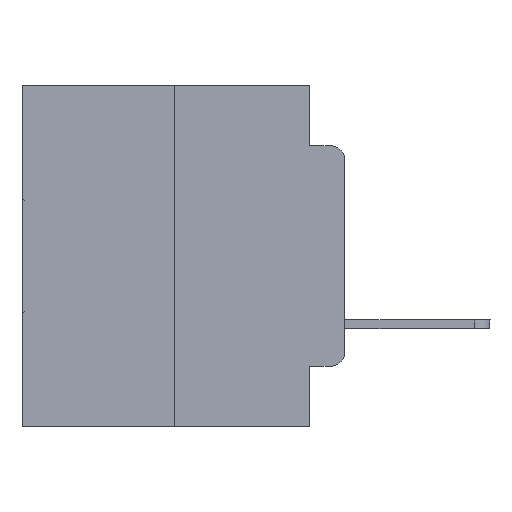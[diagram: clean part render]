
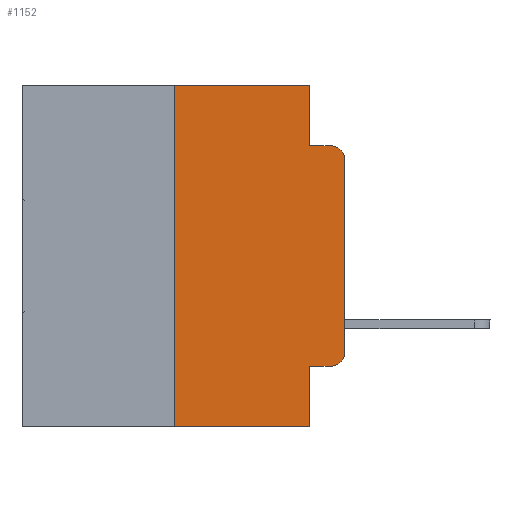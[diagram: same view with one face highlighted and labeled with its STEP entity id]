
A CAD part, left-side view. The second image highlights one B-rep face of the part: STEP entity #1152.
In plain terms, the highlighted planar face has unit normal (-1, 0, 0).
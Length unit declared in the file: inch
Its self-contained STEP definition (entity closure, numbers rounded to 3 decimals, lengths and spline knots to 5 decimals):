
#126 = CARTESIAN_POINT ( 'NONE',  ( 0., 0.051, 0. ) ) ;
#404 = EDGE_CURVE ( 'NONE', #18520, #23628, #30501, .T. ) ;
#711 = DIRECTION ( 'NONE',  ( 0., -1., 0. ) ) ;
#727 = CARTESIAN_POINT ( 'NONE',  ( 0., 0.051, -0.4115 ) ) ;
#1152 = ADVANCED_FACE ( 'NONE', ( #8216 ), #8423, .F. ) ;
#2028 = VECTOR ( 'NONE', #17372, 39.37008 ) ;
#2049 = AXIS2_PLACEMENT_3D ( 'NONE', #23591, #7626, #17096 ) ;
#3329 = VERTEX_POINT ( 'NONE', #16156 ) ;
#3701 = EDGE_CURVE ( 'NONE', #27090, #26414, #9958, .T. ) ;
#3841 = ORIENTED_EDGE ( 'NONE', *, *, #16722, .F. ) ;
#5215 = VERTEX_POINT ( 'NONE', #24459 ) ;
#5327 = ORIENTED_EDGE ( 'NONE', *, *, #24524, .T. ) ;
#6388 = CARTESIAN_POINT ( 'NONE',  ( 0., 0.051, -0.5 ) ) ;
#6832 = EDGE_LOOP ( 'NONE', ( #15181, #20966, #20983, #3841, #15462, #10433, #23345, #9398, #5327, #10752 ) ) ;
#7091 = CARTESIAN_POINT ( 'NONE',  ( 0., 0.02, -0.1085 ) ) ;
#7365 = CARTESIAN_POINT ( 'NONE',  ( 0., 0.02, -0.4115 ) ) ;
#7626 = DIRECTION ( 'NONE',  ( -1., 0., 0. ) ) ;
#8216 = FACE_OUTER_BOUND ( 'NONE', #6832, .T. ) ;
#8360 = CIRCLE ( 'NONE', #16550, 0.02 ) ;
#8423 = PLANE ( 'NONE',  #13833 ) ;
#8676 = CARTESIAN_POINT ( 'NONE',  ( 0., 0., 0. ) ) ;
#9398 = ORIENTED_EDGE ( 'NONE', *, *, #404, .F. ) ;
#9728 = LINE ( 'NONE', #727, #10491 ) ;
#9752 = CARTESIAN_POINT ( 'NONE',  ( 0., 0.051, 0. ) ) ;
#9958 = LINE ( 'NONE', #14859, #27630 ) ;
#10280 = CIRCLE ( 'NONE', #2049, 0.02 ) ;
#10433 = ORIENTED_EDGE ( 'NONE', *, *, #19518, .F. ) ;
#10491 = VECTOR ( 'NONE', #12619, 39.37008 ) ;
#10752 = ORIENTED_EDGE ( 'NONE', *, *, #28095, .T. ) ;
#11494 = LINE ( 'NONE', #26331, #2028 ) ;
#11509 = CARTESIAN_POINT ( 'NONE',  ( 0., 0.051, -0.0885 ) ) ;
#11803 = EDGE_CURVE ( 'NONE', #3329, #29284, #28330, .T. ) ;
#12619 = DIRECTION ( 'NONE',  ( 0., -1., 0. ) ) ;
#13703 = LINE ( 'NONE', #26568, #14792 ) ;
#13833 = AXIS2_PLACEMENT_3D ( 'NONE', #15436, #15740, #20057 ) ;
#14544 = DIRECTION ( 'NONE',  ( 0., -1., 0. ) ) ;
#14792 = VECTOR ( 'NONE', #14544, 39.37008 ) ;
#14859 = CARTESIAN_POINT ( 'NONE',  ( 0., 0.051, -0.0885 ) ) ;
#15181 = ORIENTED_EDGE ( 'NONE', *, *, #11803, .T. ) ;
#15436 = CARTESIAN_POINT ( 'NONE',  ( 0., 0.473, 0. ) ) ;
#15462 = ORIENTED_EDGE ( 'NONE', *, *, #20221, .F. ) ;
#15500 = VECTOR ( 'NONE', #21257, 39.37008 ) ;
#15740 = DIRECTION ( 'NONE',  ( 1., 0., 0. ) ) ;
#15881 = LINE ( 'NONE', #9752, #15500 ) ;
#16063 = CARTESIAN_POINT ( 'NONE',  ( 0., 0.02, -0.0885 ) ) ;
#16156 = CARTESIAN_POINT ( 'NONE',  ( 0., 0., -0.3915 ) ) ;
#16394 = EDGE_CURVE ( 'NONE', #19009, #23628, #11494, .T. ) ;
#16550 = AXIS2_PLACEMENT_3D ( 'NONE', #7091, #20910, #23569 ) ;
#16722 = EDGE_CURVE ( 'NONE', #17122, #27090, #15881, .T. ) ;
#17096 = DIRECTION ( 'NONE',  ( 0., 0., -1. ) ) ;
#17122 = VERTEX_POINT ( 'NONE', #25854 ) ;
#17372 = DIRECTION ( 'NONE',  ( 0., -1., 0. ) ) ;
#17491 = CARTESIAN_POINT ( 'NONE',  ( 0., 0.25, -0.5 ) ) ;
#17986 = VECTOR ( 'NONE', #24128, 39.37008 ) ;
#18520 = VERTEX_POINT ( 'NONE', #28403 ) ;
#18806 = EDGE_CURVE ( 'NONE', #29284, #26414, #8360, .T. ) ;
#19009 = VERTEX_POINT ( 'NONE', #17491 ) ;
#19091 = VECTOR ( 'NONE', #20429, 39.37008 ) ;
#19203 = CARTESIAN_POINT ( 'NONE',  ( 0., 0.25, 0. ) ) ;
#19518 = EDGE_CURVE ( 'NONE', #19009, #5215, #30045, .T. ) ;
#20057 = DIRECTION ( 'NONE',  ( 0., 0., -1. ) ) ;
#20221 = EDGE_CURVE ( 'NONE', #5215, #17122, #13703, .T. ) ;
#20429 = DIRECTION ( 'NONE',  ( 0., 0., 1. ) ) ;
#20910 = DIRECTION ( 'NONE',  ( -1., 0., 0. ) ) ;
#20966 = ORIENTED_EDGE ( 'NONE', *, *, #18806, .T. ) ;
#20983 = ORIENTED_EDGE ( 'NONE', *, *, #3701, .F. ) ;
#21257 = DIRECTION ( 'NONE',  ( 0., 0., -1. ) ) ;
#23345 = ORIENTED_EDGE ( 'NONE', *, *, #16394, .T. ) ;
#23569 = DIRECTION ( 'NONE',  ( 0., 0., -1. ) ) ;
#23591 = CARTESIAN_POINT ( 'NONE',  ( 0., 0.02, -0.3915 ) ) ;
#23628 = VERTEX_POINT ( 'NONE', #6388 ) ;
#23754 = VECTOR ( 'NONE', #24132, 39.37008 ) ;
#24128 = DIRECTION ( 'NONE',  ( 0., 0., -1. ) ) ;
#24132 = DIRECTION ( 'NONE',  ( 0., 0., 1. ) ) ;
#24459 = CARTESIAN_POINT ( 'NONE',  ( 0., 0.25, 0. ) ) ;
#24524 = EDGE_CURVE ( 'NONE', #18520, #29392, #9728, .T. ) ;
#25854 = CARTESIAN_POINT ( 'NONE',  ( 0., 0.051, 0. ) ) ;
#26331 = CARTESIAN_POINT ( 'NONE',  ( 0., 0.473, -0.5 ) ) ;
#26414 = VERTEX_POINT ( 'NONE', #16063 ) ;
#26568 = CARTESIAN_POINT ( 'NONE',  ( 0., 0.473, 0. ) ) ;
#27090 = VERTEX_POINT ( 'NONE', #11509 ) ;
#27630 = VECTOR ( 'NONE', #711, 39.37008 ) ;
#27991 = CARTESIAN_POINT ( 'NONE',  ( 0., 0., -0.1085 ) ) ;
#28095 = EDGE_CURVE ( 'NONE', #29392, #3329, #10280, .T. ) ;
#28330 = LINE ( 'NONE', #8676, #19091 ) ;
#28403 = CARTESIAN_POINT ( 'NONE',  ( 0., 0.051, -0.4115 ) ) ;
#29284 = VERTEX_POINT ( 'NONE', #27991 ) ;
#29392 = VERTEX_POINT ( 'NONE', #7365 ) ;
#30045 = LINE ( 'NONE', #19203, #23754 ) ;
#30501 = LINE ( 'NONE', #126, #17986 ) ;
